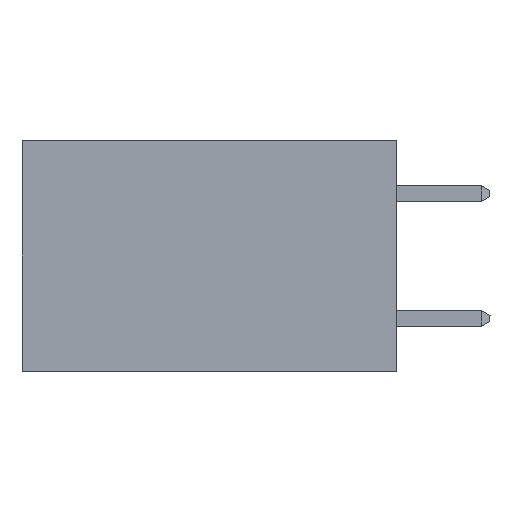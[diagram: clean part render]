
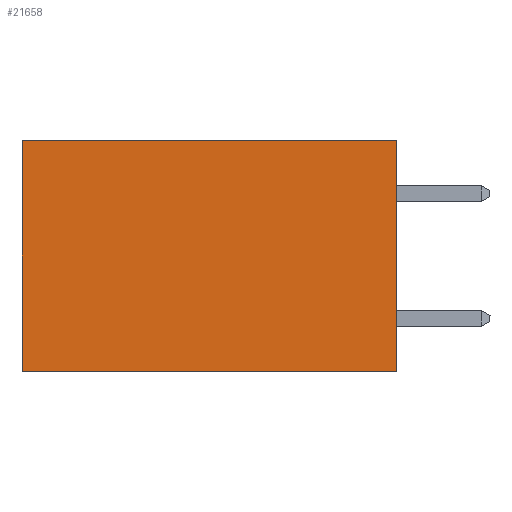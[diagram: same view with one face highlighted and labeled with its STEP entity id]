
A CAD part, left-side view. The second image highlights one B-rep face of the part: STEP entity #21658.
In plain terms, the highlighted planar face has unit normal (-1, 0, 0).
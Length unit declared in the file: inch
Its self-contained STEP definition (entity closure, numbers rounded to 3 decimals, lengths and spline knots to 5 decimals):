
#416 = VERTEX_POINT ( 'NONE', #6654 ) ;
#2175 = EDGE_CURVE ( 'NONE', #416, #11441, #7721, .T. ) ;
#2387 = FACE_OUTER_BOUND ( 'NONE', #6394, .T. ) ;
#3969 = EDGE_CURVE ( 'NONE', #14875, #11441, #9064, .T. ) ;
#4757 = PLANE ( 'NONE',  #6022 ) ;
#4825 = VECTOR ( 'NONE', #18475, 39.37008 ) ;
#5508 = VECTOR ( 'NONE', #14436, 39.37008 ) ;
#6022 = AXIS2_PLACEMENT_3D ( 'NONE', #16700, #16968, #16903 ) ;
#6189 = CARTESIAN_POINT ( 'NONE',  ( 0.298, 0., 0. ) ) ;
#6394 = EDGE_LOOP ( 'NONE', ( #9332, #19211, #21980, #8257 ) ) ;
#6654 = CARTESIAN_POINT ( 'NONE',  ( 0.298, 0., -0.37 ) ) ;
#6949 = DIRECTION ( 'NONE',  ( 0., 0., -1. ) ) ;
#7117 = EDGE_CURVE ( 'NONE', #19247, #14875, #21985, .T. ) ;
#7238 = CARTESIAN_POINT ( 'NONE',  ( 0.298, 0.6, 0. ) ) ;
#7721 = LINE ( 'NONE', #21965, #4825 ) ;
#8257 = ORIENTED_EDGE ( 'NONE', *, *, #7117, .T. ) ;
#9064 = LINE ( 'NONE', #18491, #12789 ) ;
#9332 = ORIENTED_EDGE ( 'NONE', *, *, #3969, .T. ) ;
#9822 = EDGE_CURVE ( 'NONE', #19247, #416, #11868, .T. ) ;
#11441 = VERTEX_POINT ( 'NONE', #16860 ) ;
#11446 = DIRECTION ( 'NONE',  ( 0., 1., 0. ) ) ;
#11868 = LINE ( 'NONE', #6189, #5508 ) ;
#12789 = VECTOR ( 'NONE', #6949, 39.37008 ) ;
#14436 = DIRECTION ( 'NONE',  ( 0., 0., -1. ) ) ;
#14478 = CARTESIAN_POINT ( 'NONE',  ( 0.298, 0., 0. ) ) ;
#14875 = VERTEX_POINT ( 'NONE', #7238 ) ;
#16700 = CARTESIAN_POINT ( 'NONE',  ( 0.298, 0., 0. ) ) ;
#16860 = CARTESIAN_POINT ( 'NONE',  ( 0.298, 0.6, -0.37 ) ) ;
#16903 = DIRECTION ( 'NONE',  ( 0., 0., -1. ) ) ;
#16968 = DIRECTION ( 'NONE',  ( 1., 0., 0. ) ) ;
#18475 = DIRECTION ( 'NONE',  ( 0., 1., 0. ) ) ;
#18491 = CARTESIAN_POINT ( 'NONE',  ( 0.298, 0.6, 0. ) ) ;
#18528 = VECTOR ( 'NONE', #11446, 39.37008 ) ;
#19211 = ORIENTED_EDGE ( 'NONE', *, *, #2175, .F. ) ;
#19247 = VERTEX_POINT ( 'NONE', #20111 ) ;
#20111 = CARTESIAN_POINT ( 'NONE',  ( 0.298, 0., 0. ) ) ;
#21658 = ADVANCED_FACE ( 'NONE', ( #2387 ), #4757, .F. ) ;
#21965 = CARTESIAN_POINT ( 'NONE',  ( 0.298, 0., -0.37 ) ) ;
#21980 = ORIENTED_EDGE ( 'NONE', *, *, #9822, .F. ) ;
#21985 = LINE ( 'NONE', #14478, #18528 ) ;
